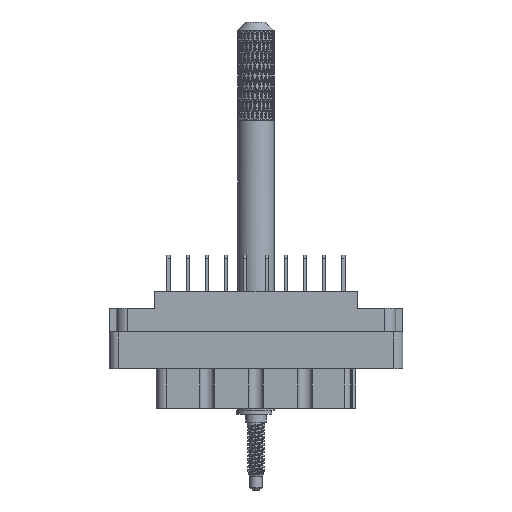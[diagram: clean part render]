
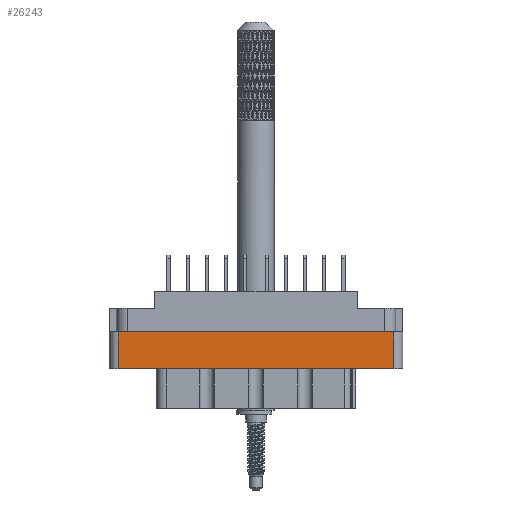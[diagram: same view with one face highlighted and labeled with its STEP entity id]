
A CAD part, front view. The second image highlights one B-rep face of the part: STEP entity #26243.
In plain terms, the highlighted planar face has unit normal (0, -1, 0).
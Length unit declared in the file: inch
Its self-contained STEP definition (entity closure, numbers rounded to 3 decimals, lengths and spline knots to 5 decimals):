
#3263 = LINE ( 'NONE', #100632, #32354 ) ;
#6235 = LINE ( 'NONE', #95155, #102767 ) ;
#8335 = EDGE_LOOP ( 'NONE', ( #100355, #39682, #43940, #71592 ) ) ;
#18275 = EDGE_CURVE ( 'NONE', #55582, #89340, #43254, .T. ) ;
#18285 = FACE_OUTER_BOUND ( 'NONE', #8335, .T. ) ;
#23694 = AXIS2_PLACEMENT_3D ( 'NONE', #35207, #65399, #41066 ) ;
#26243 = ADVANCED_FACE ( 'NONE', ( #18285 ), #90804, .T. ) ;
#26483 = LINE ( 'NONE', #84670, #49631 ) ;
#32354 = VECTOR ( 'NONE', #43475, 39.37008 ) ;
#35207 = CARTESIAN_POINT ( 'NONE',  ( -1., -0.438, -0.798 ) ) ;
#39682 = ORIENTED_EDGE ( 'NONE', *, *, #97518, .T. ) ;
#41066 = DIRECTION ( 'NONE',  ( 0., 0., -1. ) ) ;
#43254 = LINE ( 'NONE', #67590, #91872 ) ;
#43475 = DIRECTION ( 'NONE',  ( 0., 0., -1. ) ) ;
#43940 = ORIENTED_EDGE ( 'NONE', *, *, #18275, .F. ) ;
#45390 = CARTESIAN_POINT ( 'NONE',  ( -0.938, -0.438, -0.277 ) ) ;
#45927 = DIRECTION ( 'NONE',  ( 0., 0., 1. ) ) ;
#49631 = VECTOR ( 'NONE', #99523, 39.37008 ) ;
#54108 = CARTESIAN_POINT ( 'NONE',  ( -0.938, -0.438, -0.529 ) ) ;
#55582 = VERTEX_POINT ( 'NONE', #85327 ) ;
#57262 = VERTEX_POINT ( 'NONE', #45390 ) ;
#65399 = DIRECTION ( 'NONE',  ( 0., -1., 0. ) ) ;
#66635 = EDGE_CURVE ( 'NONE', #57262, #99659, #26483, .T. ) ;
#67590 = CARTESIAN_POINT ( 'NONE',  ( 0., -0.438, -0.529 ) ) ;
#71592 = ORIENTED_EDGE ( 'NONE', *, *, #89589, .T. ) ;
#74270 = CARTESIAN_POINT ( 'NONE',  ( 0.938, -0.438, -0.277 ) ) ;
#84670 = CARTESIAN_POINT ( 'NONE',  ( 0., -0.438, -0.277 ) ) ;
#85327 = CARTESIAN_POINT ( 'NONE',  ( 0.938, -0.438, -0.529 ) ) ;
#89340 = VERTEX_POINT ( 'NONE', #54108 ) ;
#89589 = EDGE_CURVE ( 'NONE', #55582, #99659, #6235, .T. ) ;
#90804 = PLANE ( 'NONE',  #23694 ) ;
#91872 = VECTOR ( 'NONE', #99887, 39.37008 ) ;
#95155 = CARTESIAN_POINT ( 'NONE',  ( 0.938, -0.438, -0.798 ) ) ;
#97518 = EDGE_CURVE ( 'NONE', #57262, #89340, #3263, .T. ) ;
#99523 = DIRECTION ( 'NONE',  ( 1., 0., 0. ) ) ;
#99659 = VERTEX_POINT ( 'NONE', #74270 ) ;
#99887 = DIRECTION ( 'NONE',  ( -1., 0., 0. ) ) ;
#100355 = ORIENTED_EDGE ( 'NONE', *, *, #66635, .F. ) ;
#100632 = CARTESIAN_POINT ( 'NONE',  ( -0.938, -0.438, -0.798 ) ) ;
#102767 = VECTOR ( 'NONE', #45927, 39.37008 ) ;
